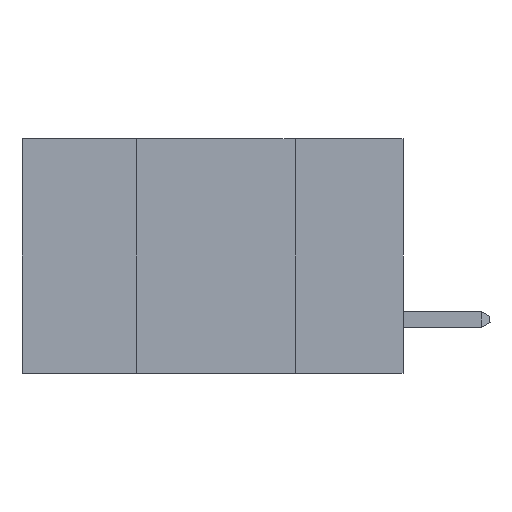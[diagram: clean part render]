
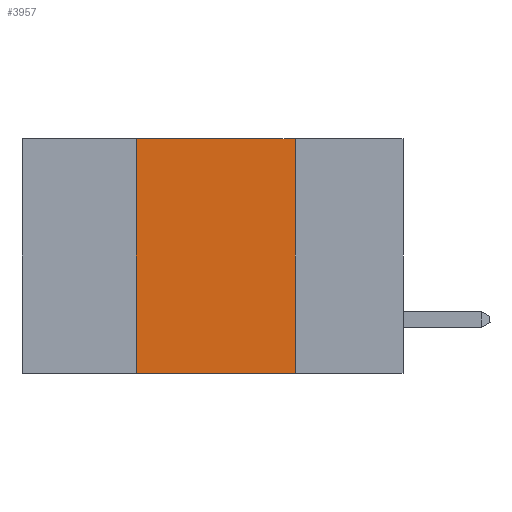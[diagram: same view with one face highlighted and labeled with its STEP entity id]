
A CAD part, left-side view. The second image highlights one B-rep face of the part: STEP entity #3957.
In plain terms, the highlighted planar face has unit normal (-1, 0, 0).
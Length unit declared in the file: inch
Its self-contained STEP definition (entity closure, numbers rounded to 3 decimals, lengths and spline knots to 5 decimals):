
#276 = CARTESIAN_POINT ( 'NONE',  ( 0., 0.17, -0.37 ) ) ;
#2502 = CARTESIAN_POINT ( 'NONE',  ( 0., 0.6, -0.37 ) ) ;
#2589 = DIRECTION ( 'NONE',  ( 0., -1., 0. ) ) ;
#3957 = ADVANCED_FACE ( 'NONE', ( #14275 ), #5764, .F. ) ;
#5321 = EDGE_CURVE ( 'NONE', #9776, #12857, #10377, .T. ) ;
#5764 = PLANE ( 'NONE',  #13357 ) ;
#6138 = EDGE_LOOP ( 'NONE', ( #17995, #17852, #25298, #8993 ) ) ;
#6453 = VECTOR ( 'NONE', #2589, 39.37008 ) ;
#7378 = CARTESIAN_POINT ( 'NONE',  ( 0., 0.42, 0. ) ) ;
#7640 = CARTESIAN_POINT ( 'NONE',  ( 0., 0.6, 0. ) ) ;
#8538 = EDGE_CURVE ( 'NONE', #13756, #18960, #14991, .T. ) ;
#8593 = EDGE_CURVE ( 'NONE', #12857, #18960, #17501, .T. ) ;
#8993 = ORIENTED_EDGE ( 'NONE', *, *, #8538, .T. ) ;
#9776 = VERTEX_POINT ( 'NONE', #14587 ) ;
#10377 = LINE ( 'NONE', #7640, #25876 ) ;
#12111 = VECTOR ( 'NONE', #12741, 39.37008 ) ;
#12741 = DIRECTION ( 'NONE',  ( 0., 0., -1. ) ) ;
#12857 = VERTEX_POINT ( 'NONE', #15880 ) ;
#13357 = AXIS2_PLACEMENT_3D ( 'NONE', #18009, #19242, #25015 ) ;
#13756 = VERTEX_POINT ( 'NONE', #14949 ) ;
#13907 = DIRECTION ( 'NONE',  ( 0., 0., 1. ) ) ;
#14275 = FACE_OUTER_BOUND ( 'NONE', #6138, .T. ) ;
#14587 = CARTESIAN_POINT ( 'NONE',  ( 0., 0.42, 0. ) ) ;
#14949 = CARTESIAN_POINT ( 'NONE',  ( 0., 0.42, -0.37 ) ) ;
#14991 = LINE ( 'NONE', #2502, #6453 ) ;
#15880 = CARTESIAN_POINT ( 'NONE',  ( 0., 0.17, 0. ) ) ;
#17501 = LINE ( 'NONE', #24872, #12111 ) ;
#17852 = ORIENTED_EDGE ( 'NONE', *, *, #5321, .F. ) ;
#17995 = ORIENTED_EDGE ( 'NONE', *, *, #8593, .F. ) ;
#18009 = CARTESIAN_POINT ( 'NONE',  ( 0., 0.6, 0. ) ) ;
#18960 = VERTEX_POINT ( 'NONE', #276 ) ;
#19242 = DIRECTION ( 'NONE',  ( 1., 0., 0. ) ) ;
#19911 = DIRECTION ( 'NONE',  ( 0., -1., 0. ) ) ;
#21658 = VECTOR ( 'NONE', #13907, 39.37008 ) ;
#24436 = EDGE_CURVE ( 'NONE', #13756, #9776, #24518, .T. ) ;
#24518 = LINE ( 'NONE', #7378, #21658 ) ;
#24872 = CARTESIAN_POINT ( 'NONE',  ( 0., 0.17, 0. ) ) ;
#25015 = DIRECTION ( 'NONE',  ( 0., 0., -1. ) ) ;
#25298 = ORIENTED_EDGE ( 'NONE', *, *, #24436, .F. ) ;
#25876 = VECTOR ( 'NONE', #19911, 39.37008 ) ;
